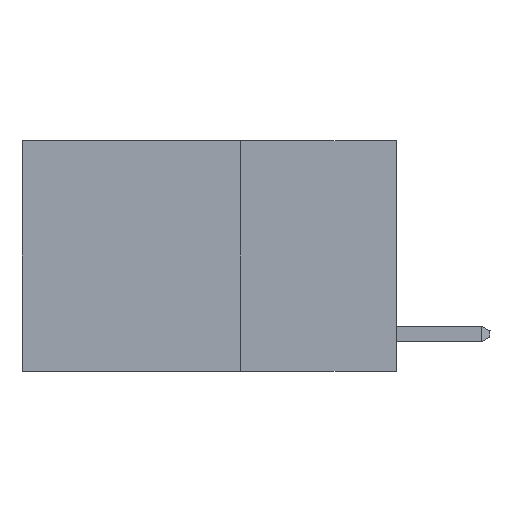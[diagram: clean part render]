
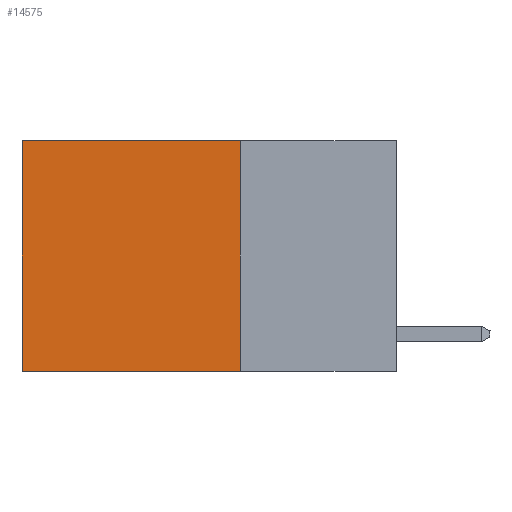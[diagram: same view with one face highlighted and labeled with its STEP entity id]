
A CAD part, left-side view. The second image highlights one B-rep face of the part: STEP entity #14575.
In plain terms, the highlighted planar face has unit normal (-1, 0, 0).
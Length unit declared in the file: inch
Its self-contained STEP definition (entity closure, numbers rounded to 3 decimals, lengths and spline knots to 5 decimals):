
#54 = VECTOR ( 'NONE', #9776, 39.37008 ) ;
#1063 = ORIENTED_EDGE ( 'NONE', *, *, #16839, .T. ) ;
#1852 = VECTOR ( 'NONE', #18294, 39.37008 ) ;
#2190 = CARTESIAN_POINT ( 'NONE',  ( 0.2625, 0.6, -0.37 ) ) ;
#2278 = VECTOR ( 'NONE', #6185, 39.37008 ) ;
#2420 = AXIS2_PLACEMENT_3D ( 'NONE', #16240, #18044, #7348 ) ;
#3338 = LINE ( 'NONE', #12259, #2278 ) ;
#4381 = ORIENTED_EDGE ( 'NONE', *, *, #5905, .T. ) ;
#4663 = LINE ( 'NONE', #17098, #14787 ) ;
#4811 = CARTESIAN_POINT ( 'NONE',  ( 0.2625, 0.25, 0. ) ) ;
#5905 = EDGE_CURVE ( 'NONE', #11314, #14566, #3338, .T. ) ;
#6001 = DIRECTION ( 'NONE',  ( 0., 1., 0. ) ) ;
#6185 = DIRECTION ( 'NONE',  ( 0., 1., 0. ) ) ;
#6534 = VERTEX_POINT ( 'NONE', #2190 ) ;
#7348 = DIRECTION ( 'NONE',  ( 0., 0., -1. ) ) ;
#8916 = CARTESIAN_POINT ( 'NONE',  ( 0.2625, 0.6, 0. ) ) ;
#9285 = EDGE_CURVE ( 'NONE', #11314, #10877, #18848, .T. ) ;
#9776 = DIRECTION ( 'NONE',  ( 0., 0., -1. ) ) ;
#9933 = LINE ( 'NONE', #8916, #1852 ) ;
#10180 = CARTESIAN_POINT ( 'NONE',  ( 0.2625, 0.6, 0. ) ) ;
#10877 = VERTEX_POINT ( 'NONE', #16772 ) ;
#11314 = VERTEX_POINT ( 'NONE', #16844 ) ;
#12259 = CARTESIAN_POINT ( 'NONE',  ( 0.2625, 0.25, 0. ) ) ;
#12290 = ORIENTED_EDGE ( 'NONE', *, *, #16458, .F. ) ;
#14095 = ORIENTED_EDGE ( 'NONE', *, *, #9285, .F. ) ;
#14566 = VERTEX_POINT ( 'NONE', #10180 ) ;
#14575 = ADVANCED_FACE ( 'NONE', ( #16340 ), #16535, .F. ) ;
#14787 = VECTOR ( 'NONE', #6001, 39.37008 ) ;
#16240 = CARTESIAN_POINT ( 'NONE',  ( 0.2625, 0.25, 0. ) ) ;
#16340 = FACE_OUTER_BOUND ( 'NONE', #18081, .T. ) ;
#16458 = EDGE_CURVE ( 'NONE', #10877, #6534, #4663, .T. ) ;
#16535 = PLANE ( 'NONE',  #2420 ) ;
#16772 = CARTESIAN_POINT ( 'NONE',  ( 0.2625, 0.25, -0.37 ) ) ;
#16839 = EDGE_CURVE ( 'NONE', #14566, #6534, #9933, .T. ) ;
#16844 = CARTESIAN_POINT ( 'NONE',  ( 0.2625, 0.25, 0. ) ) ;
#17098 = CARTESIAN_POINT ( 'NONE',  ( 0.2625, 0.25, -0.37 ) ) ;
#18044 = DIRECTION ( 'NONE',  ( 1., 0., 0. ) ) ;
#18081 = EDGE_LOOP ( 'NONE', ( #1063, #12290, #14095, #4381 ) ) ;
#18294 = DIRECTION ( 'NONE',  ( 0., 0., -1. ) ) ;
#18848 = LINE ( 'NONE', #4811, #54 ) ;
